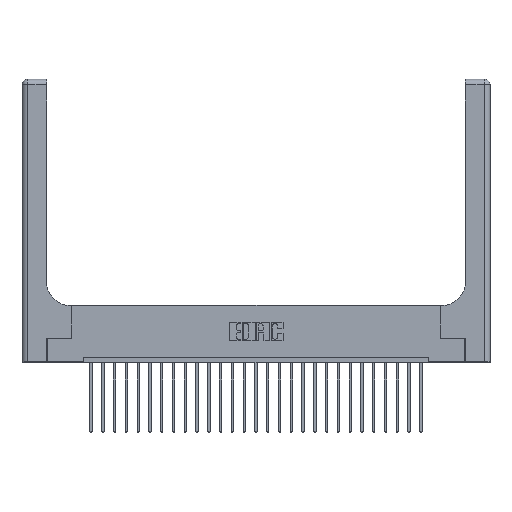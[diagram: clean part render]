
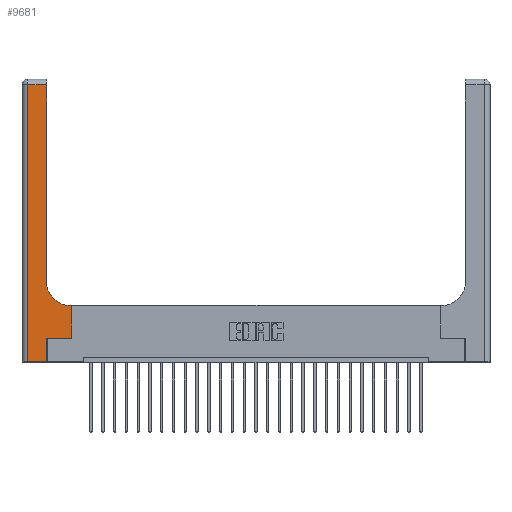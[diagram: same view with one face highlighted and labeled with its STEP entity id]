
A CAD part, top view. The second image highlights one B-rep face of the part: STEP entity #9681.
In plain terms, the highlighted planar face has unit normal (0, 0, 1).
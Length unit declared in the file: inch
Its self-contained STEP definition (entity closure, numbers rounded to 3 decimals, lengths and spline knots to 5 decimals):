
#3 = LINE ( 'NONE', #9651, #435 ) ;
#233 = VECTOR ( 'NONE', #4854, 39.37008 ) ;
#435 = VECTOR ( 'NONE', #9920, 39.37008 ) ;
#977 = CARTESIAN_POINT ( 'NONE',  ( 0.528, 0.25, 0.37 ) ) ;
#1513 = CARTESIAN_POINT ( 'NONE',  ( 0.528, 0.6, 0.37 ) ) ;
#1551 = AXIS2_PLACEMENT_3D ( 'NONE', #8402, #10578, #18386 ) ;
#1815 = DIRECTION ( 'NONE',  ( 0., -1., 0. ) ) ;
#2252 = AXIS2_PLACEMENT_3D ( 'NONE', #13162, #3626, #11491 ) ;
#2332 = ORIENTED_EDGE ( 'NONE', *, *, #18161, .T. ) ;
#2335 = EDGE_CURVE ( 'NONE', #2963, #18530, #7326, .T. ) ;
#2678 = VERTEX_POINT ( 'NONE', #15283 ) ;
#2963 = VERTEX_POINT ( 'NONE', #11044 ) ;
#3039 = ORIENTED_EDGE ( 'NONE', *, *, #9213, .T. ) ;
#3626 = DIRECTION ( 'NONE',  ( 0., 0., -1. ) ) ;
#4417 = VERTEX_POINT ( 'NONE', #977 ) ;
#4577 = VERTEX_POINT ( 'NONE', #8795 ) ;
#4597 = EDGE_CURVE ( 'NONE', #4417, #16881, #18649, .T. ) ;
#4854 = DIRECTION ( 'NONE',  ( 1., 0., 0. ) ) ;
#5061 = LINE ( 'NONE', #14701, #9009 ) ;
#6202 = VERTEX_POINT ( 'NONE', #14033 ) ;
#7099 = EDGE_CURVE ( 'NONE', #6202, #13487, #17680, .T. ) ;
#7326 = CIRCLE ( 'NONE', #1551, 0.25 ) ;
#7551 = ORIENTED_EDGE ( 'NONE', *, *, #4597, .T. ) ;
#8402 = CARTESIAN_POINT ( 'NONE',  ( 0.51, 0.85, 0.37 ) ) ;
#8795 = CARTESIAN_POINT ( 'NONE',  ( 0.265, 0.25, 0.37 ) ) ;
#9009 = VECTOR ( 'NONE', #20585, 39.37008 ) ;
#9213 = EDGE_CURVE ( 'NONE', #16881, #2963, #17171, .T. ) ;
#9487 = DIRECTION ( 'NONE',  ( -1., 0., 0. ) ) ;
#9605 = EDGE_CURVE ( 'NONE', #13487, #16968, #19165, .T. ) ;
#9651 = CARTESIAN_POINT ( 'NONE',  ( 0.265, 0., 0.37 ) ) ;
#9681 = ADVANCED_FACE ( 'NONE', ( #13536 ), #15313, .F. ) ;
#9920 = DIRECTION ( 'NONE',  ( 0., 1., 0. ) ) ;
#10247 = VECTOR ( 'NONE', #15568, 39.37008 ) ;
#10578 = DIRECTION ( 'NONE',  ( 0., 0., -1. ) ) ;
#10676 = EDGE_LOOP ( 'NONE', ( #19087, #16735, #12183, #22412, #2332, #14985, #7551, #3039, #12233 ) ) ;
#10847 = EDGE_CURVE ( 'NONE', #4577, #4417, #16648, .T. ) ;
#11044 = CARTESIAN_POINT ( 'NONE',  ( 0.51, 0.6, 0.37 ) ) ;
#11048 = VECTOR ( 'NONE', #17101, 39.37008 ) ;
#11491 = DIRECTION ( 'NONE',  ( -1., 0., 0. ) ) ;
#11607 = CARTESIAN_POINT ( 'NONE',  ( 0.06, 3., 0.37 ) ) ;
#12047 = CARTESIAN_POINT ( 'NONE',  ( 0., 2.94, 0.37 ) ) ;
#12183 = ORIENTED_EDGE ( 'NONE', *, *, #9605, .T. ) ;
#12233 = ORIENTED_EDGE ( 'NONE', *, *, #2335, .T. ) ;
#12884 = VECTOR ( 'NONE', #13975, 39.37008 ) ;
#13054 = CARTESIAN_POINT ( 'NONE',  ( 0.06, 2.94, 0.37 ) ) ;
#13162 = CARTESIAN_POINT ( 'NONE',  ( 0., 3., 0.37 ) ) ;
#13293 = VECTOR ( 'NONE', #9487, 39.37008 ) ;
#13487 = VERTEX_POINT ( 'NONE', #13054 ) ;
#13536 = FACE_OUTER_BOUND ( 'NONE', #10676, .T. ) ;
#13772 = LINE ( 'NONE', #17741, #10247 ) ;
#13975 = DIRECTION ( 'NONE',  ( -1., 0., 0. ) ) ;
#14033 = CARTESIAN_POINT ( 'NONE',  ( 0.26, 2.94, 0.37 ) ) ;
#14233 = CARTESIAN_POINT ( 'NONE',  ( 0.265, 0.25, 0.37 ) ) ;
#14701 = CARTESIAN_POINT ( 'NONE',  ( 0.26, 3., 0.37 ) ) ;
#14939 = VECTOR ( 'NONE', #1815, 39.37008 ) ;
#14985 = ORIENTED_EDGE ( 'NONE', *, *, #10847, .T. ) ;
#15092 = EDGE_CURVE ( 'NONE', #16968, #2678, #13772, .T. ) ;
#15283 = CARTESIAN_POINT ( 'NONE',  ( 0.265, 0., 0.37 ) ) ;
#15313 = PLANE ( 'NONE',  #2252 ) ;
#15568 = DIRECTION ( 'NONE',  ( 1., 0., 0. ) ) ;
#16589 = EDGE_CURVE ( 'NONE', #18530, #6202, #5061, .T. ) ;
#16648 = LINE ( 'NONE', #14233, #233 ) ;
#16735 = ORIENTED_EDGE ( 'NONE', *, *, #7099, .T. ) ;
#16881 = VERTEX_POINT ( 'NONE', #1513 ) ;
#16968 = VERTEX_POINT ( 'NONE', #17421 ) ;
#17101 = DIRECTION ( 'NONE',  ( 0., 1., 0. ) ) ;
#17171 = LINE ( 'NONE', #18853, #13293 ) ;
#17421 = CARTESIAN_POINT ( 'NONE',  ( 0.06, 0., 0.37 ) ) ;
#17680 = LINE ( 'NONE', #12047, #12884 ) ;
#17741 = CARTESIAN_POINT ( 'NONE',  ( 0., 0., 0.37 ) ) ;
#18161 = EDGE_CURVE ( 'NONE', #2678, #4577, #3, .T. ) ;
#18386 = DIRECTION ( 'NONE',  ( 1., 0., 0. ) ) ;
#18530 = VERTEX_POINT ( 'NONE', #20775 ) ;
#18649 = LINE ( 'NONE', #22990, #11048 ) ;
#18853 = CARTESIAN_POINT ( 'NONE',  ( 0.26, 0.6, 0.37 ) ) ;
#19087 = ORIENTED_EDGE ( 'NONE', *, *, #16589, .T. ) ;
#19165 = LINE ( 'NONE', #11607, #14939 ) ;
#20585 = DIRECTION ( 'NONE',  ( 0., 1., 0. ) ) ;
#20775 = CARTESIAN_POINT ( 'NONE',  ( 0.26, 0.85, 0.37 ) ) ;
#22412 = ORIENTED_EDGE ( 'NONE', *, *, #15092, .T. ) ;
#22990 = CARTESIAN_POINT ( 'NONE',  ( 0.528, 0.25, 0.37 ) ) ;
